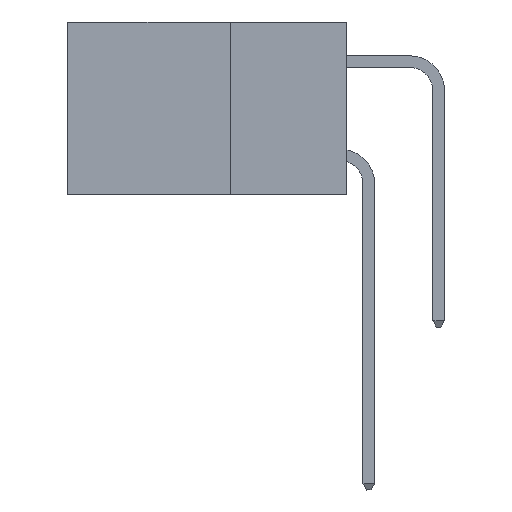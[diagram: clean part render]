
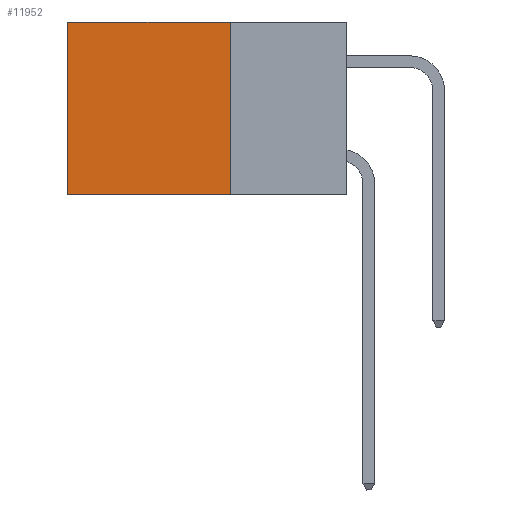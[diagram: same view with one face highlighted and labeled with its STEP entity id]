
A CAD part, left-side view. The second image highlights one B-rep face of the part: STEP entity #11952.
In plain terms, the highlighted planar face has unit normal (-1, 0, 0).
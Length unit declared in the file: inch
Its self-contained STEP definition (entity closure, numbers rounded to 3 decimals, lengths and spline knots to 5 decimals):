
#660 = CARTESIAN_POINT ( 'NONE',  ( 0.2875, 0.25, 0. ) ) ;
#1292 = VERTEX_POINT ( 'NONE', #27509 ) ;
#1807 = DIRECTION ( 'NONE',  ( 0., 1., 0. ) ) ;
#2601 = CARTESIAN_POINT ( 'NONE',  ( 0.2875, 0.25, 0. ) ) ;
#4168 = PLANE ( 'NONE',  #34326 ) ;
#5411 = VECTOR ( 'NONE', #1807, 39.37008 ) ;
#7200 = CARTESIAN_POINT ( 'NONE',  ( 0.2875, 0.6, 0. ) ) ;
#7378 = CARTESIAN_POINT ( 'NONE',  ( 0.2875, 0.25, -0.37 ) ) ;
#9607 = VECTOR ( 'NONE', #22351, 39.37008 ) ;
#9846 = ORIENTED_EDGE ( 'NONE', *, *, #13937, .F. ) ;
#11952 = ADVANCED_FACE ( 'NONE', ( #29259 ), #4168, .F. ) ;
#12189 = VECTOR ( 'NONE', #24225, 39.37008 ) ;
#12548 = CARTESIAN_POINT ( 'NONE',  ( 0.2875, 0.25, 0. ) ) ;
#13937 = EDGE_CURVE ( 'NONE', #22854, #15898, #25122, .T. ) ;
#14231 = EDGE_CURVE ( 'NONE', #22854, #21361, #25565, .T. ) ;
#15898 = VERTEX_POINT ( 'NONE', #24098 ) ;
#17418 = DIRECTION ( 'NONE',  ( 0., 0., -1. ) ) ;
#20654 = EDGE_CURVE ( 'NONE', #15898, #1292, #32386, .T. ) ;
#21361 = VERTEX_POINT ( 'NONE', #35878 ) ;
#22271 = ORIENTED_EDGE ( 'NONE', *, *, #14231, .T. ) ;
#22351 = DIRECTION ( 'NONE',  ( 0., 1., 0. ) ) ;
#22854 = VERTEX_POINT ( 'NONE', #28347 ) ;
#24098 = CARTESIAN_POINT ( 'NONE',  ( 0.2875, 0.25, -0.37 ) ) ;
#24225 = DIRECTION ( 'NONE',  ( 0., 0., -1. ) ) ;
#24586 = LINE ( 'NONE', #7200, #12189 ) ;
#25122 = LINE ( 'NONE', #660, #29975 ) ;
#25565 = LINE ( 'NONE', #2601, #9607 ) ;
#26400 = DIRECTION ( 'NONE',  ( 0., 0., -1. ) ) ;
#26681 = EDGE_LOOP ( 'NONE', ( #30962, #29446, #9846, #22271 ) ) ;
#27509 = CARTESIAN_POINT ( 'NONE',  ( 0.2875, 0.6, -0.37 ) ) ;
#28347 = CARTESIAN_POINT ( 'NONE',  ( 0.2875, 0.25, 0. ) ) ;
#29259 = FACE_OUTER_BOUND ( 'NONE', #26681, .T. ) ;
#29446 = ORIENTED_EDGE ( 'NONE', *, *, #20654, .F. ) ;
#29975 = VECTOR ( 'NONE', #17418, 39.37008 ) ;
#30962 = ORIENTED_EDGE ( 'NONE', *, *, #30971, .T. ) ;
#30971 = EDGE_CURVE ( 'NONE', #21361, #1292, #24586, .T. ) ;
#32325 = DIRECTION ( 'NONE',  ( 1., 0., 0. ) ) ;
#32386 = LINE ( 'NONE', #7378, #5411 ) ;
#34326 = AXIS2_PLACEMENT_3D ( 'NONE', #12548, #32325, #26400 ) ;
#35878 = CARTESIAN_POINT ( 'NONE',  ( 0.2875, 0.6, 0. ) ) ;
